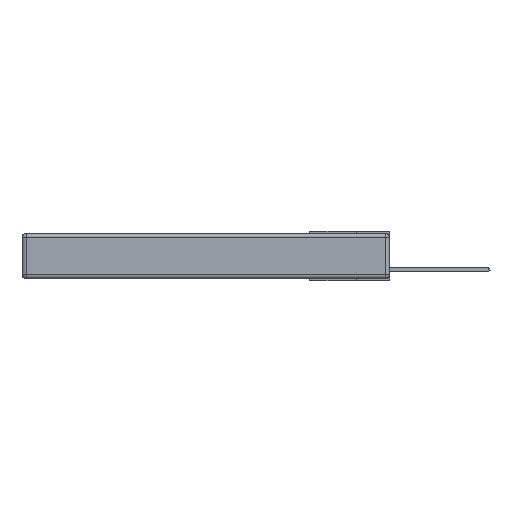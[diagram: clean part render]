
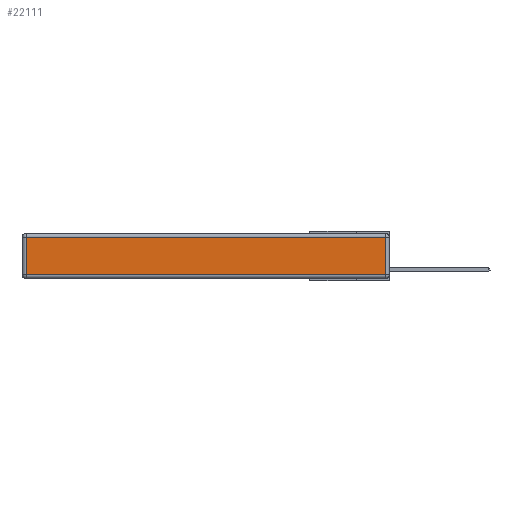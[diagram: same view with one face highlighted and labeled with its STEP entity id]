
A CAD part, left-side view. The second image highlights one B-rep face of the part: STEP entity #22111.
In plain terms, the highlighted planar face has unit normal (-1, 0, 0).
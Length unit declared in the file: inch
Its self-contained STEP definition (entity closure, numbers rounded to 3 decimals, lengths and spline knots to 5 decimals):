
#777 = CARTESIAN_POINT ( 'NONE',  ( 0., 0.03, -0.03 ) ) ;
#1165 = VERTEX_POINT ( 'NONE', #777 ) ;
#1773 = CARTESIAN_POINT ( 'NONE',  ( 0., 0.03, -0.313 ) ) ;
#4831 = DIRECTION ( 'NONE',  ( 0., 0., 1. ) ) ;
#5806 = EDGE_LOOP ( 'NONE', ( #25025, #8214, #25593, #22046 ) ) ;
#5935 = LINE ( 'NONE', #27802, #16903 ) ;
#6115 = CARTESIAN_POINT ( 'NONE',  ( 0., 2.72, -0.313 ) ) ;
#6274 = VERTEX_POINT ( 'NONE', #6115 ) ;
#6941 = PLANE ( 'NONE',  #16421 ) ;
#7724 = VECTOR ( 'NONE', #19090, 39.37008 ) ;
#7916 = CARTESIAN_POINT ( 'NONE',  ( 0., 2.72, -0.03 ) ) ;
#8214 = ORIENTED_EDGE ( 'NONE', *, *, #23256, .T. ) ;
#10345 = FACE_OUTER_BOUND ( 'NONE', #5806, .T. ) ;
#10923 = DIRECTION ( 'NONE',  ( 0., -1., 0. ) ) ;
#11288 = EDGE_CURVE ( 'NONE', #26187, #6274, #5935, .T. ) ;
#11473 = CARTESIAN_POINT ( 'NONE',  ( 0., 0., -0.343 ) ) ;
#12266 = CARTESIAN_POINT ( 'NONE',  ( 0., 0.03, -0.343 ) ) ;
#13197 = EDGE_CURVE ( 'NONE', #6274, #25575, #16595, .T. ) ;
#13302 = LINE ( 'NONE', #12266, #17079 ) ;
#13912 = LINE ( 'NONE', #27992, #7724 ) ;
#15375 = CARTESIAN_POINT ( 'NONE',  ( 0., 0., -0.313 ) ) ;
#16421 = AXIS2_PLACEMENT_3D ( 'NONE', #11473, #24830, #4831 ) ;
#16595 = LINE ( 'NONE', #15375, #19304 ) ;
#16903 = VECTOR ( 'NONE', #18723, 39.37008 ) ;
#17079 = VECTOR ( 'NONE', #21133, 39.37008 ) ;
#18169 = EDGE_CURVE ( 'NONE', #1165, #26187, #13912, .T. ) ;
#18723 = DIRECTION ( 'NONE',  ( 0., 0., -1. ) ) ;
#19090 = DIRECTION ( 'NONE',  ( 0., 1., 0. ) ) ;
#19304 = VECTOR ( 'NONE', #10923, 39.37008 ) ;
#21133 = DIRECTION ( 'NONE',  ( 0., 0., 1. ) ) ;
#22046 = ORIENTED_EDGE ( 'NONE', *, *, #11288, .T. ) ;
#22111 = ADVANCED_FACE ( 'NONE', ( #10345 ), #6941, .T. ) ;
#23256 = EDGE_CURVE ( 'NONE', #25575, #1165, #13302, .T. ) ;
#24830 = DIRECTION ( 'NONE',  ( -1., 0., 0. ) ) ;
#25025 = ORIENTED_EDGE ( 'NONE', *, *, #13197, .T. ) ;
#25575 = VERTEX_POINT ( 'NONE', #1773 ) ;
#25593 = ORIENTED_EDGE ( 'NONE', *, *, #18169, .T. ) ;
#26187 = VERTEX_POINT ( 'NONE', #7916 ) ;
#27802 = CARTESIAN_POINT ( 'NONE',  ( 0., 2.72, -0.343 ) ) ;
#27992 = CARTESIAN_POINT ( 'NONE',  ( 0., 2.75, -0.03 ) ) ;
